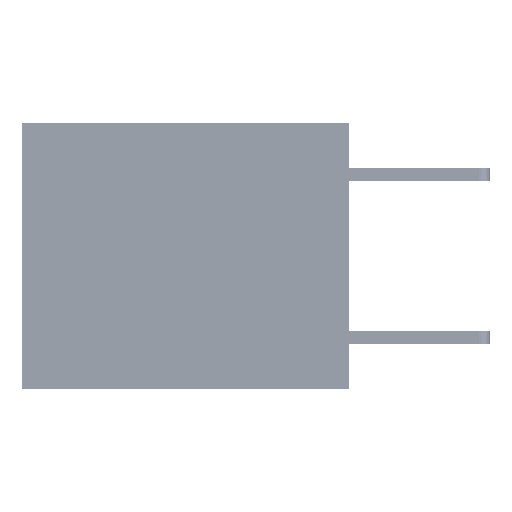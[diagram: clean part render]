
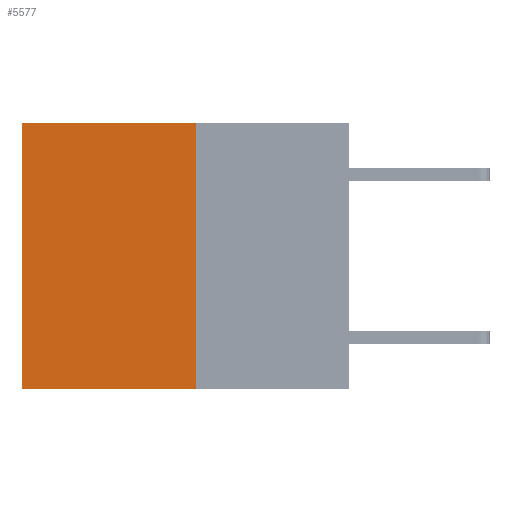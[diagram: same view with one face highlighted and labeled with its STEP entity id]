
A CAD part, left-side view. The second image highlights one B-rep face of the part: STEP entity #5577.
In plain terms, the highlighted planar face has unit normal (-1, 0, 0).
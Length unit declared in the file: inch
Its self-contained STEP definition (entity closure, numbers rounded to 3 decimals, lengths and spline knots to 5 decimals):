
#504 = EDGE_CURVE ( 'NONE', #25789, #23085, #29032, .T. ) ;
#822 = EDGE_CURVE ( 'NONE', #23085, #23004, #12525, .T. ) ;
#2204 = DIRECTION ( 'NONE',  ( 0., 1., 0. ) ) ;
#2289 = FACE_OUTER_BOUND ( 'NONE', #9624, .T. ) ;
#4425 = CARTESIAN_POINT ( 'NONE',  ( 0.3165, 0.28, -0.49 ) ) ;
#5487 = ORIENTED_EDGE ( 'NONE', *, *, #504, .T. ) ;
#5577 = ADVANCED_FACE ( 'NONE', ( #2289 ), #24134, .F. ) ;
#5896 = CARTESIAN_POINT ( 'NONE',  ( 0.3165, 0.6, 0. ) ) ;
#7608 = CARTESIAN_POINT ( 'NONE',  ( 0.3165, 0.28, -0.49 ) ) ;
#9299 = LINE ( 'NONE', #26585, #15349 ) ;
#9624 = EDGE_LOOP ( 'NONE', ( #11351, #17354, #33145, #5487 ) ) ;
#10367 = DIRECTION ( 'NONE',  ( 1., 0., 0. ) ) ;
#10755 = AXIS2_PLACEMENT_3D ( 'NONE', #7608, #10367, #28267 ) ;
#11008 = VECTOR ( 'NONE', #24892, 39.37008 ) ;
#11083 = EDGE_CURVE ( 'NONE', #25789, #34092, #34813, .T. ) ;
#11351 = ORIENTED_EDGE ( 'NONE', *, *, #822, .T. ) ;
#12525 = LINE ( 'NONE', #28463, #22437 ) ;
#14701 = VECTOR ( 'NONE', #2204, 39.37008 ) ;
#15349 = VECTOR ( 'NONE', #18335, 39.37008 ) ;
#17354 = ORIENTED_EDGE ( 'NONE', *, *, #27217, .F. ) ;
#18152 = CARTESIAN_POINT ( 'NONE',  ( 0.3165, 0.28, 0. ) ) ;
#18335 = DIRECTION ( 'NONE',  ( 0., 1., 0. ) ) ;
#22437 = VECTOR ( 'NONE', #25558, 39.37008 ) ;
#23004 = VERTEX_POINT ( 'NONE', #32503 ) ;
#23085 = VERTEX_POINT ( 'NONE', #5896 ) ;
#24134 = PLANE ( 'NONE',  #10755 ) ;
#24892 = DIRECTION ( 'NONE',  ( 0., 0., -1. ) ) ;
#25558 = DIRECTION ( 'NONE',  ( 0., 0., -1. ) ) ;
#25789 = VERTEX_POINT ( 'NONE', #30793 ) ;
#26585 = CARTESIAN_POINT ( 'NONE',  ( 0.3165, 0.28, -0.49 ) ) ;
#27217 = EDGE_CURVE ( 'NONE', #34092, #23004, #9299, .T. ) ;
#28267 = DIRECTION ( 'NONE',  ( 0., 0., -1. ) ) ;
#28463 = CARTESIAN_POINT ( 'NONE',  ( 0.3165, 0.6, -0.49 ) ) ;
#29032 = LINE ( 'NONE', #18152, #14701 ) ;
#30111 = CARTESIAN_POINT ( 'NONE',  ( 0.3165, 0.28, -0.49 ) ) ;
#30793 = CARTESIAN_POINT ( 'NONE',  ( 0.3165, 0.28, 0. ) ) ;
#32503 = CARTESIAN_POINT ( 'NONE',  ( 0.3165, 0.6, -0.49 ) ) ;
#33145 = ORIENTED_EDGE ( 'NONE', *, *, #11083, .F. ) ;
#34092 = VERTEX_POINT ( 'NONE', #4425 ) ;
#34813 = LINE ( 'NONE', #30111, #11008 ) ;
